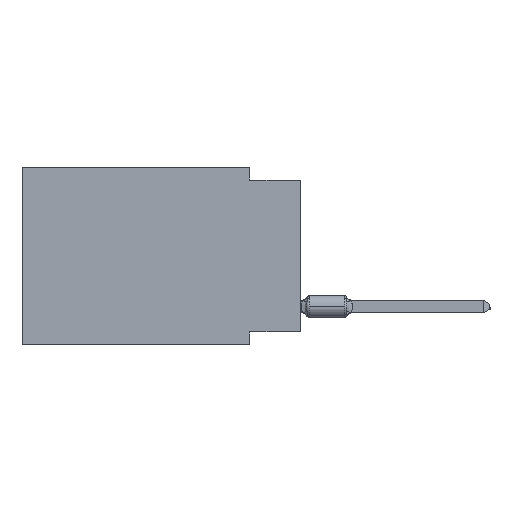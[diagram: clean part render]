
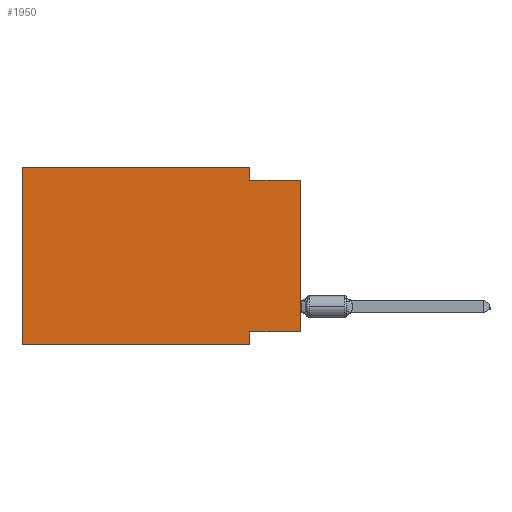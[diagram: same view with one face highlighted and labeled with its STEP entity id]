
A CAD part, left-side view. The second image highlights one B-rep face of the part: STEP entity #1950.
In plain terms, the highlighted planar face has unit normal (-1, 0, 0).
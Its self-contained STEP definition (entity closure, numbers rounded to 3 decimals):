
#290 = VERTEX_POINT ( 'NONE', #59081 ) ;
#1002 = LINE ( 'NONE', #18161, #17037 ) ;
#1894 = AXIS2_PLACEMENT_3D ( 'NONE', #51261, #62285, #34495 ) ;
#1950 = ADVANCED_FACE ( 'NONE', ( #13351 ), #23564, .F. ) ;
#4907 = VECTOR ( 'NONE', #71871, 1000. ) ;
#6067 = ORIENTED_EDGE ( 'NONE', *, *, #58980, .F. ) ;
#6654 = ORIENTED_EDGE ( 'NONE', *, *, #41058, .F. ) ;
#6945 = LINE ( 'NONE', #46698, #36613 ) ;
#9201 = VERTEX_POINT ( 'NONE', #50012 ) ;
#9209 = DIRECTION ( 'NONE',  ( 0., -1., 0. ) ) ;
#9401 = CARTESIAN_POINT ( 'NONE',  ( 0., 13.97, -8.89 ) ) ;
#11538 = EDGE_CURVE ( 'NONE', #37243, #30328, #1002, .T. ) ;
#12819 = VECTOR ( 'NONE', #46720, 1000. ) ;
#13145 = VECTOR ( 'NONE', #71988, 1000. ) ;
#13297 = VERTEX_POINT ( 'NONE', #65031 ) ;
#13351 = FACE_OUTER_BOUND ( 'NONE', #69857, .T. ) ;
#14366 = LINE ( 'NONE', #59213, #35151 ) ;
#17037 = VECTOR ( 'NONE', #40399, 1000. ) ;
#17321 = LINE ( 'NONE', #24578, #31483 ) ;
#18161 = CARTESIAN_POINT ( 'NONE',  ( 0., 13.97, 0. ) ) ;
#19856 = LINE ( 'NONE', #44157, #13145 ) ;
#21941 = CARTESIAN_POINT ( 'NONE',  ( 0., 13.97, -8.89 ) ) ;
#22680 = CARTESIAN_POINT ( 'NONE',  ( 0., 0., -8.255 ) ) ;
#23564 = PLANE ( 'NONE',  #1894 ) ;
#24578 = CARTESIAN_POINT ( 'NONE',  ( 0., 0., 0. ) ) ;
#25662 = ORIENTED_EDGE ( 'NONE', *, *, #39664, .T. ) ;
#27251 = EDGE_CURVE ( 'NONE', #9201, #57288, #17321, .T. ) ;
#28529 = ORIENTED_EDGE ( 'NONE', *, *, #44302, .F. ) ;
#30328 = VERTEX_POINT ( 'NONE', #54549 ) ;
#31483 = VECTOR ( 'NONE', #51927, 1000. ) ;
#34495 = DIRECTION ( 'NONE',  ( 0., 0., -1. ) ) ;
#35151 = VECTOR ( 'NONE', #9209, 1000. ) ;
#35524 = CARTESIAN_POINT ( 'NONE',  ( 0., 0., -0.635 ) ) ;
#35910 = ORIENTED_EDGE ( 'NONE', *, *, #27251, .T. ) ;
#36150 = LINE ( 'NONE', #52570, #12819 ) ;
#36613 = VECTOR ( 'NONE', #69059, 1000. ) ;
#36966 = ORIENTED_EDGE ( 'NONE', *, *, #11538, .F. ) ;
#37243 = VERTEX_POINT ( 'NONE', #21941 ) ;
#39295 = EDGE_CURVE ( 'NONE', #54330, #57288, #14366, .T. ) ;
#39664 = EDGE_CURVE ( 'NONE', #37243, #48695, #60485, .T. ) ;
#40246 = CARTESIAN_POINT ( 'NONE',  ( 0., 2.54, -8.89 ) ) ;
#40399 = DIRECTION ( 'NONE',  ( 0., 0., 1. ) ) ;
#41058 = EDGE_CURVE ( 'NONE', #290, #54330, #6945, .T. ) ;
#44157 = CARTESIAN_POINT ( 'NONE',  ( 0., 2.54, -8.89 ) ) ;
#44302 = EDGE_CURVE ( 'NONE', #9201, #13297, #56595, .T. ) ;
#46698 = CARTESIAN_POINT ( 'NONE',  ( 0., 2.54, 0. ) ) ;
#46720 = DIRECTION ( 'NONE',  ( 0., -1., 0. ) ) ;
#48695 = VERTEX_POINT ( 'NONE', #40246 ) ;
#50012 = CARTESIAN_POINT ( 'NONE',  ( 0., 0., -8.255 ) ) ;
#51261 = CARTESIAN_POINT ( 'NONE',  ( 0., 13.97, 0. ) ) ;
#51927 = DIRECTION ( 'NONE',  ( 0., 0., 1. ) ) ;
#52570 = CARTESIAN_POINT ( 'NONE',  ( 0., 13.97, 0. ) ) ;
#54330 = VERTEX_POINT ( 'NONE', #62341 ) ;
#54549 = CARTESIAN_POINT ( 'NONE',  ( 0., 13.97, 0. ) ) ;
#56246 = DIRECTION ( 'NONE',  ( 0., 1., 0. ) ) ;
#56595 = LINE ( 'NONE', #22680, #68605 ) ;
#56838 = ORIENTED_EDGE ( 'NONE', *, *, #69657, .F. ) ;
#57288 = VERTEX_POINT ( 'NONE', #35524 ) ;
#58558 = ORIENTED_EDGE ( 'NONE', *, *, #39295, .F. ) ;
#58980 = EDGE_CURVE ( 'NONE', #30328, #290, #36150, .T. ) ;
#59081 = CARTESIAN_POINT ( 'NONE',  ( 0., 2.54, 0. ) ) ;
#59213 = CARTESIAN_POINT ( 'NONE',  ( 0., 0., -0.635 ) ) ;
#60485 = LINE ( 'NONE', #9401, #4907 ) ;
#62285 = DIRECTION ( 'NONE',  ( 1., 0., 0. ) ) ;
#62341 = CARTESIAN_POINT ( 'NONE',  ( 0., 2.54, -0.635 ) ) ;
#65031 = CARTESIAN_POINT ( 'NONE',  ( 0., 2.54, -8.255 ) ) ;
#68605 = VECTOR ( 'NONE', #56246, 1000. ) ;
#69059 = DIRECTION ( 'NONE',  ( 0., 0., -1. ) ) ;
#69657 = EDGE_CURVE ( 'NONE', #13297, #48695, #19856, .T. ) ;
#69857 = EDGE_LOOP ( 'NONE', ( #35910, #58558, #6654, #6067, #36966, #25662, #56838, #28529 ) ) ;
#71871 = DIRECTION ( 'NONE',  ( 0., -1., 0. ) ) ;
#71988 = DIRECTION ( 'NONE',  ( 0., 0., -1. ) ) ;
